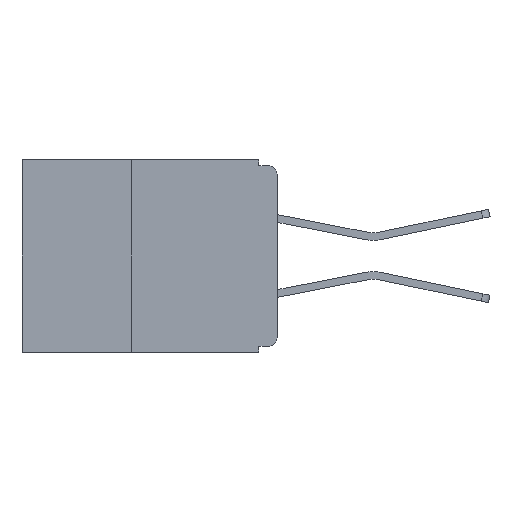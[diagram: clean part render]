
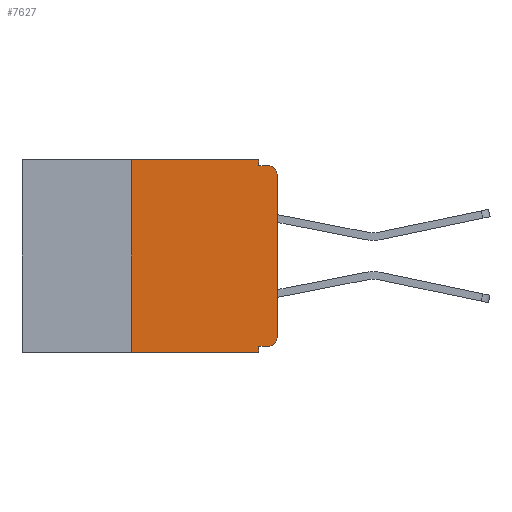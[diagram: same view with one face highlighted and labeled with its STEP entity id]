
A CAD part, left-side view. The second image highlights one B-rep face of the part: STEP entity #7627.
In plain terms, the highlighted planar face has unit normal (-1, 0, 0).
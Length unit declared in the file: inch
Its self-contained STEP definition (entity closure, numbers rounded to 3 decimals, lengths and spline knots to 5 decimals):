
#224 = ORIENTED_EDGE ( 'NONE', *, *, #20202, .T. ) ;
#417 = DIRECTION ( 'NONE',  ( -1., 0., 0. ) ) ;
#589 = CARTESIAN_POINT ( 'NONE',  ( 0., 0.015, -0.025 ) ) ;
#864 = LINE ( 'NONE', #4102, #10654 ) ;
#2291 = CARTESIAN_POINT ( 'NONE',  ( 0., 0.015, -0.01 ) ) ;
#2493 = DIRECTION ( 'NONE',  ( 0., 0., -1. ) ) ;
#3005 = DIRECTION ( 'NONE',  ( 0., -1., 0. ) ) ;
#3080 = VECTOR ( 'NONE', #18607, 39.37008 ) ;
#3164 = DIRECTION ( 'NONE',  ( 1., 0., 0. ) ) ;
#3455 = EDGE_CURVE ( 'NONE', #22424, #9542, #8317, .T. ) ;
#4102 = CARTESIAN_POINT ( 'NONE',  ( 0., 0., -0.32 ) ) ;
#4143 = VECTOR ( 'NONE', #5262, 39.37008 ) ;
#4737 = LINE ( 'NONE', #24757, #4143 ) ;
#5030 = CARTESIAN_POINT ( 'NONE',  ( 0., 0.437, 0. ) ) ;
#5262 = DIRECTION ( 'NONE',  ( 0., -1., 0. ) ) ;
#5269 = VERTEX_POINT ( 'NONE', #7579 ) ;
#5564 = CARTESIAN_POINT ( 'NONE',  ( 0., 0., -0.01 ) ) ;
#5649 = CARTESIAN_POINT ( 'NONE',  ( 0., 0.031, -0.33 ) ) ;
#6958 = CARTESIAN_POINT ( 'NONE',  ( 0., 0., -0.305 ) ) ;
#7579 = CARTESIAN_POINT ( 'NONE',  ( 0., 0., -0.025 ) ) ;
#7627 = ADVANCED_FACE ( 'NONE', ( #24904 ), #24608, .F. ) ;
#7791 = ORIENTED_EDGE ( 'NONE', *, *, #8823, .T. ) ;
#8114 = ORIENTED_EDGE ( 'NONE', *, *, #9194, .F. ) ;
#8136 = AXIS2_PLACEMENT_3D ( 'NONE', #589, #14268, #2493 ) ;
#8317 = LINE ( 'NONE', #20785, #3080 ) ;
#8823 = EDGE_CURVE ( 'NONE', #5269, #13311, #20440, .T. ) ;
#8841 = CARTESIAN_POINT ( 'NONE',  ( 0., 0.437, -0.33 ) ) ;
#9033 = CIRCLE ( 'NONE', #15731, 0.015 ) ;
#9194 = EDGE_CURVE ( 'NONE', #18005, #13311, #16156, .T. ) ;
#9542 = VERTEX_POINT ( 'NONE', #12846 ) ;
#9590 = VECTOR ( 'NONE', #21345, 39.37008 ) ;
#9841 = EDGE_CURVE ( 'NONE', #19660, #18005, #11848, .T. ) ;
#10330 = CARTESIAN_POINT ( 'NONE',  ( 0., 0.031, -0.33 ) ) ;
#10654 = VECTOR ( 'NONE', #19800, 39.37008 ) ;
#10684 = VERTEX_POINT ( 'NONE', #10330 ) ;
#10833 = LINE ( 'NONE', #5649, #9590 ) ;
#11250 = ORIENTED_EDGE ( 'NONE', *, *, #9841, .F. ) ;
#11471 = ORIENTED_EDGE ( 'NONE', *, *, #21401, .F. ) ;
#11589 = VECTOR ( 'NONE', #17320, 39.37008 ) ;
#11829 = ORIENTED_EDGE ( 'NONE', *, *, #3455, .F. ) ;
#11848 = LINE ( 'NONE', #13718, #21027 ) ;
#12125 = CARTESIAN_POINT ( 'NONE',  ( 0., 0.015, -0.305 ) ) ;
#12377 = ORIENTED_EDGE ( 'NONE', *, *, #18594, .T. ) ;
#12430 = ORIENTED_EDGE ( 'NONE', *, *, #22694, .F. ) ;
#12452 = ORIENTED_EDGE ( 'NONE', *, *, #18969, .F. ) ;
#12647 = ORIENTED_EDGE ( 'NONE', *, *, #20191, .T. ) ;
#12846 = CARTESIAN_POINT ( 'NONE',  ( 0., 0.25, 0. ) ) ;
#12904 = VERTEX_POINT ( 'NONE', #6958 ) ;
#13311 = VERTEX_POINT ( 'NONE', #2291 ) ;
#13345 = AXIS2_PLACEMENT_3D ( 'NONE', #5030, #3164, #16876 ) ;
#13647 = VECTOR ( 'NONE', #16046, 39.37008 ) ;
#13718 = CARTESIAN_POINT ( 'NONE',  ( 0., 0.031, 0. ) ) ;
#14096 = DIRECTION ( 'NONE',  ( 0., 0., -1. ) ) ;
#14268 = DIRECTION ( 'NONE',  ( -1., 0., 0. ) ) ;
#14697 = CARTESIAN_POINT ( 'NONE',  ( 0., 0.25, -0.33 ) ) ;
#14962 = CARTESIAN_POINT ( 'NONE',  ( 0., 0.031, -0.01 ) ) ;
#15280 = LINE ( 'NONE', #8841, #24388 ) ;
#15731 = AXIS2_PLACEMENT_3D ( 'NONE', #12125, #417, #14096 ) ;
#16046 = DIRECTION ( 'NONE',  ( 0., 0., 1. ) ) ;
#16156 = LINE ( 'NONE', #5564, #11589 ) ;
#16876 = DIRECTION ( 'NONE',  ( 0., 0., -1. ) ) ;
#16986 = VERTEX_POINT ( 'NONE', #23920 ) ;
#17320 = DIRECTION ( 'NONE',  ( 0., -1., 0. ) ) ;
#18005 = VERTEX_POINT ( 'NONE', #14962 ) ;
#18594 = EDGE_CURVE ( 'NONE', #22424, #10684, #15280, .T. ) ;
#18607 = DIRECTION ( 'NONE',  ( 0., 0., 1. ) ) ;
#18856 = LINE ( 'NONE', #21872, #13647 ) ;
#18969 = EDGE_CURVE ( 'NONE', #16986, #19193, #864, .T. ) ;
#19193 = VERTEX_POINT ( 'NONE', #22340 ) ;
#19660 = VERTEX_POINT ( 'NONE', #22067 ) ;
#19800 = DIRECTION ( 'NONE',  ( 0., 1., 0. ) ) ;
#20191 = EDGE_CURVE ( 'NONE', #16986, #12904, #9033, .T. ) ;
#20202 = EDGE_CURVE ( 'NONE', #12904, #5269, #18856, .T. ) ;
#20440 = CIRCLE ( 'NONE', #8136, 0.015 ) ;
#20785 = CARTESIAN_POINT ( 'NONE',  ( 0., 0.25, -0.33 ) ) ;
#21027 = VECTOR ( 'NONE', #21576, 39.37008 ) ;
#21345 = DIRECTION ( 'NONE',  ( 0., 0., -1. ) ) ;
#21401 = EDGE_CURVE ( 'NONE', #9542, #19660, #4737, .T. ) ;
#21576 = DIRECTION ( 'NONE',  ( 0., 0., -1. ) ) ;
#21872 = CARTESIAN_POINT ( 'NONE',  ( 0., 0., 0. ) ) ;
#22067 = CARTESIAN_POINT ( 'NONE',  ( 0., 0.031, 0. ) ) ;
#22103 = EDGE_LOOP ( 'NONE', ( #224, #7791, #8114, #11250, #11471, #11829, #12377, #12430, #12452, #12647 ) ) ;
#22340 = CARTESIAN_POINT ( 'NONE',  ( 0., 0.031, -0.32 ) ) ;
#22424 = VERTEX_POINT ( 'NONE', #14697 ) ;
#22694 = EDGE_CURVE ( 'NONE', #19193, #10684, #10833, .T. ) ;
#23920 = CARTESIAN_POINT ( 'NONE',  ( 0., 0.015, -0.32 ) ) ;
#24388 = VECTOR ( 'NONE', #3005, 39.37008 ) ;
#24608 = PLANE ( 'NONE',  #13345 ) ;
#24757 = CARTESIAN_POINT ( 'NONE',  ( 0., 0.437, 0. ) ) ;
#24904 = FACE_OUTER_BOUND ( 'NONE', #22103, .T. ) ;
